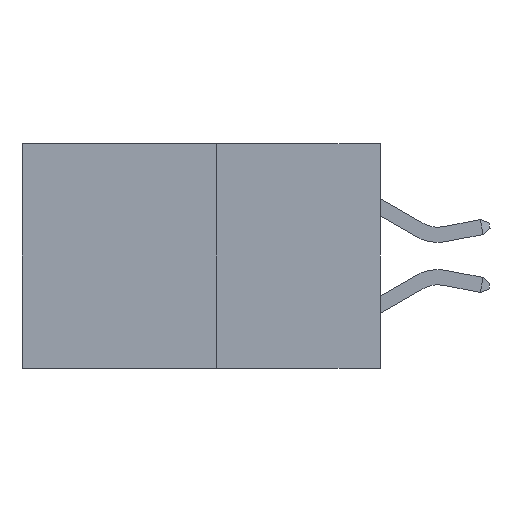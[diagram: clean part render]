
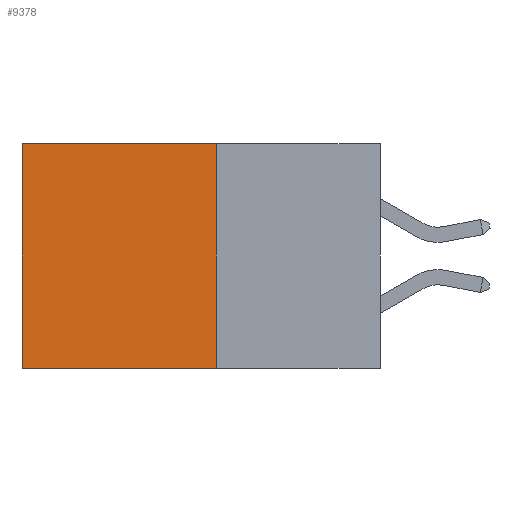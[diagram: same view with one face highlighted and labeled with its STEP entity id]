
A CAD part, left-side view. The second image highlights one B-rep face of the part: STEP entity #9378.
In plain terms, the highlighted planar face has unit normal (-1, 0, 0).
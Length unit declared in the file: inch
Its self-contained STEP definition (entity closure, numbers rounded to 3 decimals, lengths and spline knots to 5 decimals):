
#515 = CARTESIAN_POINT ( 'NONE',  ( 0.277, 0.27, -0.37 ) ) ;
#652 = CARTESIAN_POINT ( 'NONE',  ( 0.277, 0.27, -0.37 ) ) ;
#734 = CARTESIAN_POINT ( 'NONE',  ( 0.277, 0.27, -0.37 ) ) ;
#1505 = DIRECTION ( 'NONE',  ( 0., 0., -1. ) ) ;
#1589 = EDGE_CURVE ( 'NONE', #8170, #8831, #5438, .T. ) ;
#1720 = CARTESIAN_POINT ( 'NONE',  ( 0.277, 0.59, 0. ) ) ;
#1884 = VERTEX_POINT ( 'NONE', #9168 ) ;
#2175 = FACE_OUTER_BOUND ( 'NONE', #2990, .T. ) ;
#2315 = DIRECTION ( 'NONE',  ( 0., 0., -1. ) ) ;
#2419 = LINE ( 'NONE', #734, #8427 ) ;
#2425 = LINE ( 'NONE', #7827, #6140 ) ;
#2990 = EDGE_LOOP ( 'NONE', ( #6426, #6496, #9021, #6998 ) ) ;
#3379 = AXIS2_PLACEMENT_3D ( 'NONE', #652, #6278, #1505 ) ;
#4758 = VECTOR ( 'NONE', #6139, 39.37008 ) ;
#5205 = CARTESIAN_POINT ( 'NONE',  ( 0.277, 0.27, 0. ) ) ;
#5438 = LINE ( 'NONE', #9835, #9537 ) ;
#5528 = DIRECTION ( 'NONE',  ( 0., 1., 0. ) ) ;
#5796 = CARTESIAN_POINT ( 'NONE',  ( 0.277, 0.59, -0.37 ) ) ;
#5829 = EDGE_CURVE ( 'NONE', #8170, #1884, #6914, .T. ) ;
#5932 = DIRECTION ( 'NONE',  ( 0., 1., 0. ) ) ;
#6139 = DIRECTION ( 'NONE',  ( 0., 0., -1. ) ) ;
#6140 = VECTOR ( 'NONE', #2315, 39.37008 ) ;
#6273 = VERTEX_POINT ( 'NONE', #5796 ) ;
#6278 = DIRECTION ( 'NONE',  ( 1., 0., 0. ) ) ;
#6426 = ORIENTED_EDGE ( 'NONE', *, *, #9399, .T. ) ;
#6496 = ORIENTED_EDGE ( 'NONE', *, *, #6717, .F. ) ;
#6717 = EDGE_CURVE ( 'NONE', #1884, #6273, #2419, .T. ) ;
#6914 = LINE ( 'NONE', #515, #4758 ) ;
#6998 = ORIENTED_EDGE ( 'NONE', *, *, #1589, .T. ) ;
#7792 = PLANE ( 'NONE',  #3379 ) ;
#7827 = CARTESIAN_POINT ( 'NONE',  ( 0.277, 0.59, -0.37 ) ) ;
#8170 = VERTEX_POINT ( 'NONE', #5205 ) ;
#8427 = VECTOR ( 'NONE', #5528, 39.37008 ) ;
#8831 = VERTEX_POINT ( 'NONE', #1720 ) ;
#9021 = ORIENTED_EDGE ( 'NONE', *, *, #5829, .F. ) ;
#9168 = CARTESIAN_POINT ( 'NONE',  ( 0.277, 0.27, -0.37 ) ) ;
#9378 = ADVANCED_FACE ( 'NONE', ( #2175 ), #7792, .F. ) ;
#9399 = EDGE_CURVE ( 'NONE', #8831, #6273, #2425, .T. ) ;
#9537 = VECTOR ( 'NONE', #5932, 39.37008 ) ;
#9835 = CARTESIAN_POINT ( 'NONE',  ( 0.277, 0.27, 0. ) ) ;
